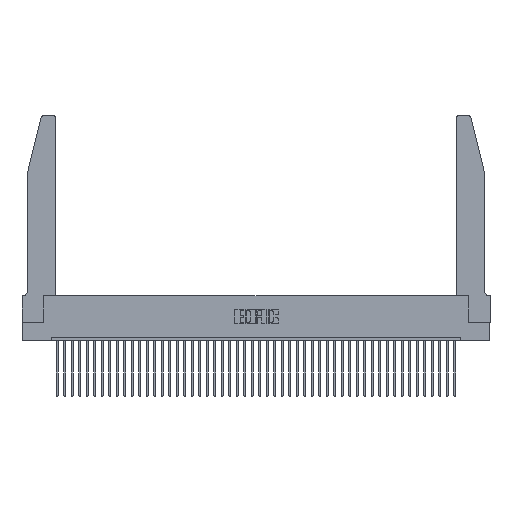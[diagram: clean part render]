
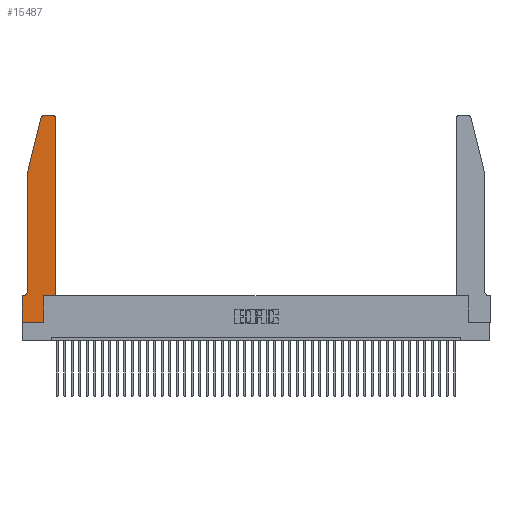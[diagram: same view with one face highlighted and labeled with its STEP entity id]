
A CAD part, top view. The second image highlights one B-rep face of the part: STEP entity #15487.
In plain terms, the highlighted planar face has unit normal (0, 0, 1).
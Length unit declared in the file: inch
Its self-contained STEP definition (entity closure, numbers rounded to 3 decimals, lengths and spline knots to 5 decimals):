
#1282 = VERTEX_POINT ( 'NONE', #21465 ) ;
#1460 = ORIENTED_EDGE ( 'NONE', *, *, #37722, .T. ) ;
#1600 = VERTEX_POINT ( 'NONE', #32726 ) ;
#1601 = CARTESIAN_POINT ( 'NONE',  ( 0., 0., 0.37 ) ) ;
#2155 = VERTEX_POINT ( 'NONE', #3958 ) ;
#2368 = VERTEX_POINT ( 'NONE', #14433 ) ;
#3958 = CARTESIAN_POINT ( 'NONE',  ( 0.25487, 2.72718, 0.37 ) ) ;
#4168 = LINE ( 'NONE', #19987, #23213 ) ;
#4685 = CARTESIAN_POINT ( 'NONE',  ( 0., 0., 0.37 ) ) ;
#4745 = ORIENTED_EDGE ( 'NONE', *, *, #6480, .T. ) ;
#5692 = AXIS2_PLACEMENT_3D ( 'NONE', #11328, #34950, #7971 ) ;
#5775 = VECTOR ( 'NONE', #8660, 39.37008 ) ;
#6116 = DIRECTION ( 'NONE',  ( 0., 1., 0. ) ) ;
#6338 = VECTOR ( 'NONE', #29646, 39.37008 ) ;
#6361 = LINE ( 'NONE', #33498, #38024 ) ;
#6480 = EDGE_CURVE ( 'NONE', #1600, #1282, #37044, .T. ) ;
#7332 = DIRECTION ( 'NONE',  ( -1., 0., 0. ) ) ;
#7506 = EDGE_CURVE ( 'NONE', #2155, #42794, #30076, .T. ) ;
#7948 = CARTESIAN_POINT ( 'NONE',  ( 0.0755, 2., 0.37 ) ) ;
#7971 = DIRECTION ( 'NONE',  ( 1., 0., 0. ) ) ;
#8043 = DIRECTION ( 'NONE',  ( 1., 0., 0. ) ) ;
#8116 = ORIENTED_EDGE ( 'NONE', *, *, #32646, .T. ) ;
#8248 = VERTEX_POINT ( 'NONE', #22183 ) ;
#8645 = VECTOR ( 'NONE', #30521, 39.37008 ) ;
#8660 = DIRECTION ( 'NONE',  ( 1., 0., 0. ) ) ;
#10097 = DIRECTION ( 'NONE',  ( -1., 0., 0. ) ) ;
#11039 = ORIENTED_EDGE ( 'NONE', *, *, #20734, .T. ) ;
#11328 = CARTESIAN_POINT ( 'NONE',  ( 0.4205, 2.72, 0.37 ) ) ;
#11675 = LINE ( 'NONE', #11906, #41807 ) ;
#11906 = CARTESIAN_POINT ( 'NONE',  ( 0.4505, 0.35, 0.37 ) ) ;
#12332 = DIRECTION ( 'NONE',  ( 0., 1., 0. ) ) ;
#13577 = CARTESIAN_POINT ( 'NONE',  ( 0.4205, 2.75, 0.37 ) ) ;
#13916 = ORIENTED_EDGE ( 'NONE', *, *, #7506, .T. ) ;
#14433 = CARTESIAN_POINT ( 'NONE',  ( 0.0755, 0.42, 0.37 ) ) ;
#14803 = VECTOR ( 'NONE', #7332, 39.37008 ) ;
#15196 = DIRECTION ( 'NONE',  ( 1., 0., 0. ) ) ;
#15487 = ADVANCED_FACE ( 'NONE', ( #25023 ), #18949, .T. ) ;
#15948 = ORIENTED_EDGE ( 'NONE', *, *, #43051, .T. ) ;
#17884 = ORIENTED_EDGE ( 'NONE', *, *, #41481, .T. ) ;
#18191 = DIRECTION ( 'NONE',  ( 0., 0., -1. ) ) ;
#18666 = CARTESIAN_POINT ( 'NONE',  ( 0.4505, 0.35, 0.37 ) ) ;
#18949 = PLANE ( 'NONE',  #35779 ) ;
#19234 = CARTESIAN_POINT ( 'NONE',  ( 0., 0.35, 0.37 ) ) ;
#19483 = LINE ( 'NONE', #18666, #5775 ) ;
#19987 = CARTESIAN_POINT ( 'NONE',  ( 0.2605, 2.75, 0.37 ) ) ;
#20734 = EDGE_CURVE ( 'NONE', #33242, #35586, #4168, .T. ) ;
#21465 = CARTESIAN_POINT ( 'NONE',  ( 0., 0.35, 0.37 ) ) ;
#21788 = VERTEX_POINT ( 'NONE', #29634 ) ;
#22169 = CARTESIAN_POINT ( 'NONE',  ( 0.2865, 0.35, 0.37 ) ) ;
#22183 = CARTESIAN_POINT ( 'NONE',  ( 0.4505, 0.35, 0.37 ) ) ;
#22703 = CARTESIAN_POINT ( 'NONE',  ( 0.0755, 2., 0.37 ) ) ;
#22802 = DIRECTION ( 'NONE',  ( 1., 0., 0. ) ) ;
#23213 = VECTOR ( 'NONE', #10097, 39.37008 ) ;
#23330 = ORIENTED_EDGE ( 'NONE', *, *, #25798, .T. ) ;
#23998 = CARTESIAN_POINT ( 'NONE',  ( 0.284, 2.75, 0.37 ) ) ;
#24242 = EDGE_LOOP ( 'NONE', ( #11039, #23330, #13916, #28719, #1460, #4745, #8116, #29400, #28694, #35247, #15948, #17884 ) ) ;
#24575 = DIRECTION ( 'NONE',  ( 0., 0., 1. ) ) ;
#24844 = EDGE_CURVE ( 'NONE', #42873, #26792, #36648, .T. ) ;
#25023 = FACE_OUTER_BOUND ( 'NONE', #24242, .T. ) ;
#25798 = EDGE_CURVE ( 'NONE', #35586, #2155, #39246, .T. ) ;
#26033 = VERTEX_POINT ( 'NONE', #22169 ) ;
#26604 = VECTOR ( 'NONE', #15196, 39.37008 ) ;
#26655 = CIRCLE ( 'NONE', #5692, 0.03 ) ;
#26792 = VERTEX_POINT ( 'NONE', #33063 ) ;
#27115 = CARTESIAN_POINT ( 'NONE',  ( 0., 0., 0.37 ) ) ;
#27506 = CARTESIAN_POINT ( 'NONE',  ( 0.0755, 0.35, 0.37 ) ) ;
#28694 = ORIENTED_EDGE ( 'NONE', *, *, #37935, .T. ) ;
#28719 = ORIENTED_EDGE ( 'NONE', *, *, #30657, .T. ) ;
#28812 = CARTESIAN_POINT ( 'NONE',  ( 0.0055, 0.42, 0.37 ) ) ;
#29400 = ORIENTED_EDGE ( 'NONE', *, *, #24844, .T. ) ;
#29634 = CARTESIAN_POINT ( 'NONE',  ( 0.4505, 2.72, 0.37 ) ) ;
#29646 = DIRECTION ( 'NONE',  ( -0.239, -0.971, 0. ) ) ;
#30076 = LINE ( 'NONE', #22703, #6338 ) ;
#30521 = DIRECTION ( 'NONE',  ( 0., -1., 0. ) ) ;
#30657 = EDGE_CURVE ( 'NONE', #42794, #2368, #6361, .T. ) ;
#31046 = EDGE_CURVE ( 'NONE', #26033, #8248, #19483, .T. ) ;
#31055 = AXIS2_PLACEMENT_3D ( 'NONE', #38472, #24575, #8043 ) ;
#32646 = EDGE_CURVE ( 'NONE', #1282, #42873, #37177, .T. ) ;
#32726 = CARTESIAN_POINT ( 'NONE',  ( 0.0055, 0.35, 0.37 ) ) ;
#32993 = LINE ( 'NONE', #40090, #40434 ) ;
#33063 = CARTESIAN_POINT ( 'NONE',  ( 0.2865, 0., 0.37 ) ) ;
#33242 = VERTEX_POINT ( 'NONE', #13577 ) ;
#33498 = CARTESIAN_POINT ( 'NONE',  ( 0.0755, 2., 0.37 ) ) ;
#34441 = AXIS2_PLACEMENT_3D ( 'NONE', #28812, #18191, #39052 ) ;
#34950 = DIRECTION ( 'NONE',  ( 0., 0., 1. ) ) ;
#35247 = ORIENTED_EDGE ( 'NONE', *, *, #31046, .T. ) ;
#35586 = VERTEX_POINT ( 'NONE', #23998 ) ;
#35779 = AXIS2_PLACEMENT_3D ( 'NONE', #19234, #39666, #22802 ) ;
#36648 = LINE ( 'NONE', #1601, #26604 ) ;
#37044 = LINE ( 'NONE', #27506, #14803 ) ;
#37177 = LINE ( 'NONE', #27115, #8645 ) ;
#37644 = DIRECTION ( 'NONE',  ( 0., -1., 0. ) ) ;
#37722 = EDGE_CURVE ( 'NONE', #2368, #1600, #42537, .T. ) ;
#37935 = EDGE_CURVE ( 'NONE', #26792, #26033, #32993, .T. ) ;
#38024 = VECTOR ( 'NONE', #37644, 39.37008 ) ;
#38472 = CARTESIAN_POINT ( 'NONE',  ( 0.284, 2.72, 0.37 ) ) ;
#39052 = DIRECTION ( 'NONE',  ( -1., 0., 0. ) ) ;
#39246 = CIRCLE ( 'NONE', #31055, 0.03 ) ;
#39666 = DIRECTION ( 'NONE',  ( 0., 0., 1. ) ) ;
#40090 = CARTESIAN_POINT ( 'NONE',  ( 0.2865, 0.35, 0.37 ) ) ;
#40434 = VECTOR ( 'NONE', #6116, 39.37008 ) ;
#41481 = EDGE_CURVE ( 'NONE', #21788, #33242, #26655, .T. ) ;
#41807 = VECTOR ( 'NONE', #12332, 39.37008 ) ;
#42537 = CIRCLE ( 'NONE', #34441, 0.07 ) ;
#42794 = VERTEX_POINT ( 'NONE', #7948 ) ;
#42873 = VERTEX_POINT ( 'NONE', #4685 ) ;
#43051 = EDGE_CURVE ( 'NONE', #8248, #21788, #11675, .T. ) ;
